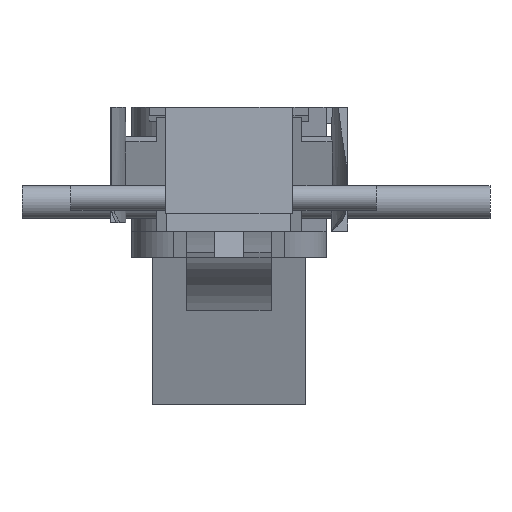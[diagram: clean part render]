
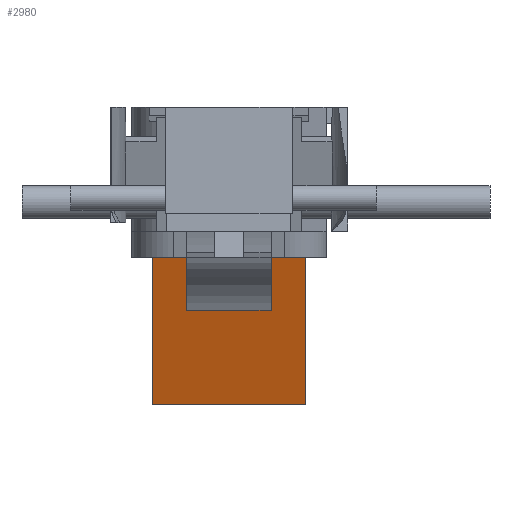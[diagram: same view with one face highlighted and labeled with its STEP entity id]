
A CAD part, left-side view. The second image highlights one B-rep face of the part: STEP entity #2980.
In plain terms, the highlighted planar face has unit normal (-0.951, 0, -0.309).
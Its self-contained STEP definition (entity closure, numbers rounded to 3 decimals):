
#189=FACE_OUTER_BOUND('',#351,.T.);
#351=EDGE_LOOP('',(#2127,#2128,#2129,#2130,#2131,#2132,#2133,#2134,#2135,
#2136));
#491=LINE('',#4067,#841);
#500=LINE('',#4087,#850);
#506=LINE('',#4111,#856);
#550=LINE('',#4201,#900);
#597=LINE('',#4888,#947);
#599=LINE('',#4892,#949);
#600=LINE('',#4893,#950);
#601=LINE('',#4894,#951);
#602=LINE('',#4896,#952);
#603=LINE('',#4897,#953);
#841=VECTOR('',#3326,10.);
#850=VECTOR('',#3341,10.);
#856=VECTOR('',#3357,1.015);
#900=VECTOR('',#3405,10.);
#947=VECTOR('',#3500,1.015);
#949=VECTOR('',#3504,10.);
#950=VECTOR('',#3505,10.);
#951=VECTOR('',#3506,10.);
#952=VECTOR('',#3507,1.015);
#953=VECTOR('',#3508,1.015);
#1189=VERTEX_POINT('',#4061);
#1191=VERTEX_POINT('',#4065);
#1198=VERTEX_POINT('',#4084);
#1199=VERTEX_POINT('',#4086);
#1206=VERTEX_POINT('',#4110);
#1249=VERTEX_POINT('',#4198);
#1250=VERTEX_POINT('',#4200);
#1300=VERTEX_POINT('',#4887);
#1301=VERTEX_POINT('',#4891);
#1302=VERTEX_POINT('',#4895);
#1487=EDGE_CURVE('',#1189,#1191,#491,.T.);
#1496=EDGE_CURVE('',#1198,#1199,#500,.T.);
#1505=EDGE_CURVE('',#1199,#1206,#506,.T.);
#1550=EDGE_CURVE('',#1249,#1250,#550,.T.);
#1621=EDGE_CURVE('',#1300,#1189,#597,.T.);
#1623=EDGE_CURVE('',#1191,#1301,#599,.T.);
#1624=EDGE_CURVE('',#1301,#1206,#600,.T.);
#1625=EDGE_CURVE('',#1198,#1250,#601,.T.);
#1626=EDGE_CURVE('',#1249,#1302,#602,.T.);
#1627=EDGE_CURVE('',#1300,#1302,#603,.T.);
#2127=ORIENTED_EDGE('',*,*,#1621,.T.);
#2128=ORIENTED_EDGE('',*,*,#1487,.T.);
#2129=ORIENTED_EDGE('',*,*,#1623,.T.);
#2130=ORIENTED_EDGE('',*,*,#1624,.T.);
#2131=ORIENTED_EDGE('',*,*,#1505,.F.);
#2132=ORIENTED_EDGE('',*,*,#1496,.F.);
#2133=ORIENTED_EDGE('',*,*,#1625,.T.);
#2134=ORIENTED_EDGE('',*,*,#1550,.F.);
#2135=ORIENTED_EDGE('',*,*,#1626,.T.);
#2136=ORIENTED_EDGE('',*,*,#1627,.F.);
#2845=PLANE('',#3159);
#2980=ADVANCED_FACE('',(#189),#2845,.T.);
#3159=AXIS2_PLACEMENT_3D('',#4890,#3502,#3503);
#3326=DIRECTION('',(0.,1.,0.));
#3341=DIRECTION('',(0.,1.,0.));
#3357=DIRECTION('',(-0.309,0.,0.951));
#3405=DIRECTION('',(0.,-1.,0.));
#3500=DIRECTION('',(0.309,0.,-0.951));
#3502=DIRECTION('center_axis',(-0.951,0.,
-0.309));
#3503=DIRECTION('ref_axis',(0.,1.,0.));
#3504=DIRECTION('',(-0.309,0.,0.951));
#3505=DIRECTION('',(0.,1.,0.));
#3506=DIRECTION('',(-0.309,0.,0.951));
#3507=DIRECTION('',(0.309,0.,-0.951));
#3508=DIRECTION('',(0.,-1.,0.));
#4061=CARTESIAN_POINT('',(-0.965,-245.692,87.658));
#4065=CARTESIAN_POINT('',(-0.965,-243.662,87.658));
#4067=CARTESIAN_POINT('',(-0.965,-272.247,87.658));
#4084=CARTESIAN_POINT('',(4.915,-260.664,69.562));
#4086=CARTESIAN_POINT('',(4.915,-241.886,69.562));
#4087=CARTESIAN_POINT('',(4.915,-272.887,69.562));
#4110=CARTESIAN_POINT('',(-3.198,-241.886,94.531));
#4111=CARTESIAN_POINT('',(5.13,-241.886,68.898));
#4198=CARTESIAN_POINT('',(-6.958,-246.454,106.102));
#4200=CARTESIAN_POINT('',(-6.958,-260.664,106.102));
#4201=CARTESIAN_POINT('',(-6.958,-263.277,106.102));
#4887=CARTESIAN_POINT('',(-3.198,-245.692,94.531));
#4888=CARTESIAN_POINT('',(2.652,-245.692,76.527));
#4890=CARTESIAN_POINT('Origin',(5.13,-260.664,68.898));
#4891=CARTESIAN_POINT('',(-3.198,-243.662,94.531));
#4892=CARTESIAN_POINT('',(1.18,-243.662,81.056));
#4893=CARTESIAN_POINT('',(-3.198,-255.886,94.531));
#4894=CARTESIAN_POINT('',(1.18,-260.664,81.056));
#4895=CARTESIAN_POINT('',(-3.198,-246.454,94.531));
#4896=CARTESIAN_POINT('',(-1.81,-246.454,90.259));
#4897=CARTESIAN_POINT('',(-3.198,-246.979,94.531));
